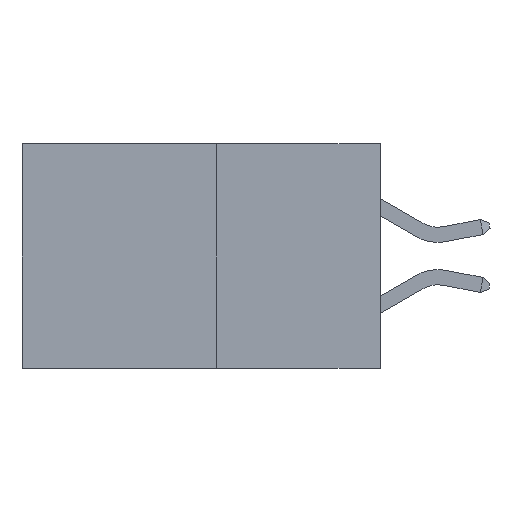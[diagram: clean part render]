
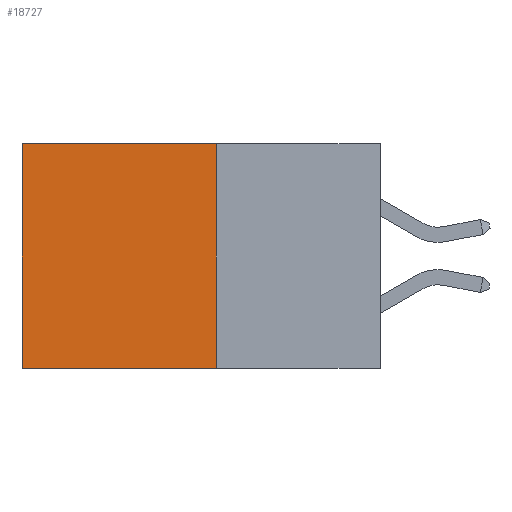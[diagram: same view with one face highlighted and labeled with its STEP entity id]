
A CAD part, left-side view. The second image highlights one B-rep face of the part: STEP entity #18727.
In plain terms, the highlighted planar face has unit normal (-1, 0, 0).
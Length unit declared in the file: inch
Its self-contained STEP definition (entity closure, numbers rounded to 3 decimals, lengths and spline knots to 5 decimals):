
#225 = EDGE_CURVE ( 'NONE', #4602, #25641, #10185, .T. ) ;
#1503 = CARTESIAN_POINT ( 'NONE',  ( 0.277, 0.27, -0.37 ) ) ;
#2895 = LINE ( 'NONE', #17220, #21987 ) ;
#3051 = LINE ( 'NONE', #27741, #15254 ) ;
#4144 = DIRECTION ( 'NONE',  ( 0., 1., 0. ) ) ;
#4269 = DIRECTION ( 'NONE',  ( 0., 0., -1. ) ) ;
#4602 = VERTEX_POINT ( 'NONE', #1503 ) ;
#5555 = VERTEX_POINT ( 'NONE', #31818 ) ;
#5843 = CARTESIAN_POINT ( 'NONE',  ( 0.277, 0.27, -0.37 ) ) ;
#10033 = ORIENTED_EDGE ( 'NONE', *, *, #18124, .T. ) ;
#10185 = LINE ( 'NONE', #5843, #10996 ) ;
#10996 = VECTOR ( 'NONE', #4144, 39.37008 ) ;
#12069 = VECTOR ( 'NONE', #21548, 39.37008 ) ;
#12366 = DIRECTION ( 'NONE',  ( 0., 0., -1. ) ) ;
#12811 = CARTESIAN_POINT ( 'NONE',  ( 0.277, 0.59, -0.37 ) ) ;
#14137 = CARTESIAN_POINT ( 'NONE',  ( 0.277, 0.27, -0.37 ) ) ;
#14880 = EDGE_LOOP ( 'NONE', ( #10033, #19777, #22019, #28309 ) ) ;
#15254 = VECTOR ( 'NONE', #12366, 39.37008 ) ;
#16728 = DIRECTION ( 'NONE',  ( 0., 0., -1. ) ) ;
#17220 = CARTESIAN_POINT ( 'NONE',  ( 0.277, 0.59, -0.37 ) ) ;
#17951 = AXIS2_PLACEMENT_3D ( 'NONE', #14137, #32000, #16728 ) ;
#18124 = EDGE_CURVE ( 'NONE', #26164, #25641, #2895, .T. ) ;
#18727 = ADVANCED_FACE ( 'NONE', ( #31452 ), #26888, .F. ) ;
#18941 = CARTESIAN_POINT ( 'NONE',  ( 0.277, 0.27, 0. ) ) ;
#19777 = ORIENTED_EDGE ( 'NONE', *, *, #225, .F. ) ;
#21195 = EDGE_CURVE ( 'NONE', #5555, #26164, #31678, .T. ) ;
#21548 = DIRECTION ( 'NONE',  ( 0., 1., 0. ) ) ;
#21987 = VECTOR ( 'NONE', #4269, 39.37008 ) ;
#22019 = ORIENTED_EDGE ( 'NONE', *, *, #30271, .F. ) ;
#22836 = CARTESIAN_POINT ( 'NONE',  ( 0.277, 0.59, 0. ) ) ;
#25641 = VERTEX_POINT ( 'NONE', #12811 ) ;
#26164 = VERTEX_POINT ( 'NONE', #22836 ) ;
#26888 = PLANE ( 'NONE',  #17951 ) ;
#27741 = CARTESIAN_POINT ( 'NONE',  ( 0.277, 0.27, -0.37 ) ) ;
#28309 = ORIENTED_EDGE ( 'NONE', *, *, #21195, .T. ) ;
#30271 = EDGE_CURVE ( 'NONE', #5555, #4602, #3051, .T. ) ;
#31452 = FACE_OUTER_BOUND ( 'NONE', #14880, .T. ) ;
#31678 = LINE ( 'NONE', #18941, #12069 ) ;
#31818 = CARTESIAN_POINT ( 'NONE',  ( 0.277, 0.27, 0. ) ) ;
#32000 = DIRECTION ( 'NONE',  ( 1., 0., 0. ) ) ;
